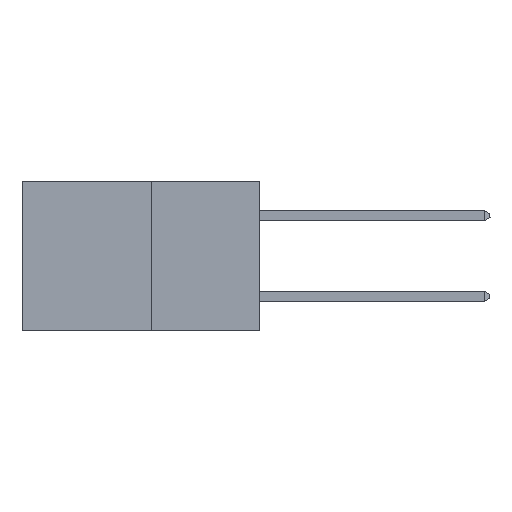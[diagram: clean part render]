
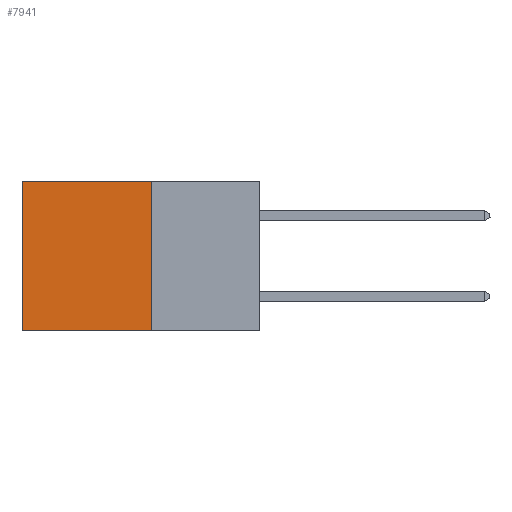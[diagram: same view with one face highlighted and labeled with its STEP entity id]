
A CAD part, left-side view. The second image highlights one B-rep face of the part: STEP entity #7941.
In plain terms, the highlighted planar face has unit normal (-1, 0, 0).
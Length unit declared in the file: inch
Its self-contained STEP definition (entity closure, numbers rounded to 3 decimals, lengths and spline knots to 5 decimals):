
#1034 = DIRECTION ( 'NONE',  ( 0., 0., -1. ) ) ;
#1597 = VECTOR ( 'NONE', #31883, 39.37008 ) ;
#2541 = DIRECTION ( 'NONE',  ( 0., 1., 0. ) ) ;
#3891 = VERTEX_POINT ( 'NONE', #9783 ) ;
#5310 = ORIENTED_EDGE ( 'NONE', *, *, #21648, .T. ) ;
#6119 = CARTESIAN_POINT ( 'NONE',  ( 0.277, 0.27, -0.37 ) ) ;
#6624 = LINE ( 'NONE', #7635, #13249 ) ;
#7635 = CARTESIAN_POINT ( 'NONE',  ( 0.277, 0.27, -0.37 ) ) ;
#7860 = VECTOR ( 'NONE', #1034, 39.37008 ) ;
#7941 = ADVANCED_FACE ( 'NONE', ( #16972 ), #28539, .F. ) ;
#8501 = CARTESIAN_POINT ( 'NONE',  ( 0.277, 0.59, -0.37 ) ) ;
#8633 = LINE ( 'NONE', #8501, #7860 ) ;
#9783 = CARTESIAN_POINT ( 'NONE',  ( 0.277, 0.59, 0. ) ) ;
#11315 = ORIENTED_EDGE ( 'NONE', *, *, #24556, .T. ) ;
#11933 = EDGE_CURVE ( 'NONE', #15150, #12949, #6624, .T. ) ;
#12597 = EDGE_LOOP ( 'NONE', ( #5310, #18827, #31914, #11315 ) ) ;
#12949 = VERTEX_POINT ( 'NONE', #31021 ) ;
#13249 = VECTOR ( 'NONE', #2541, 39.37008 ) ;
#13660 = DIRECTION ( 'NONE',  ( 1., 0., 0. ) ) ;
#14901 = LINE ( 'NONE', #29409, #1597 ) ;
#15150 = VERTEX_POINT ( 'NONE', #15683 ) ;
#15683 = CARTESIAN_POINT ( 'NONE',  ( 0.277, 0.27, -0.37 ) ) ;
#15710 = VECTOR ( 'NONE', #26767, 39.37008 ) ;
#16513 = LINE ( 'NONE', #24273, #15710 ) ;
#16972 = FACE_OUTER_BOUND ( 'NONE', #12597, .T. ) ;
#17959 = VERTEX_POINT ( 'NONE', #29359 ) ;
#18827 = ORIENTED_EDGE ( 'NONE', *, *, #11933, .F. ) ;
#20018 = EDGE_CURVE ( 'NONE', #17959, #15150, #16513, .T. ) ;
#21648 = EDGE_CURVE ( 'NONE', #3891, #12949, #8633, .T. ) ;
#24273 = CARTESIAN_POINT ( 'NONE',  ( 0.277, 0.27, -0.37 ) ) ;
#24556 = EDGE_CURVE ( 'NONE', #17959, #3891, #14901, .T. ) ;
#26767 = DIRECTION ( 'NONE',  ( 0., 0., -1. ) ) ;
#28539 = PLANE ( 'NONE',  #29037 ) ;
#29037 = AXIS2_PLACEMENT_3D ( 'NONE', #6119, #13660, #31023 ) ;
#29359 = CARTESIAN_POINT ( 'NONE',  ( 0.277, 0.27, 0. ) ) ;
#29409 = CARTESIAN_POINT ( 'NONE',  ( 0.277, 0.27, 0. ) ) ;
#31021 = CARTESIAN_POINT ( 'NONE',  ( 0.277, 0.59, -0.37 ) ) ;
#31023 = DIRECTION ( 'NONE',  ( 0., 0., -1. ) ) ;
#31883 = DIRECTION ( 'NONE',  ( 0., 1., 0. ) ) ;
#31914 = ORIENTED_EDGE ( 'NONE', *, *, #20018, .F. ) ;
